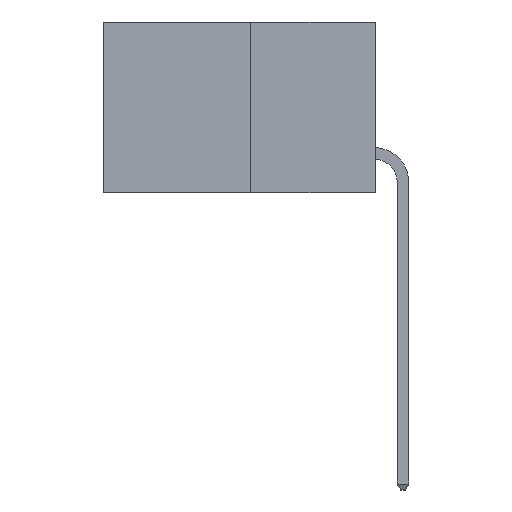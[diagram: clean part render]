
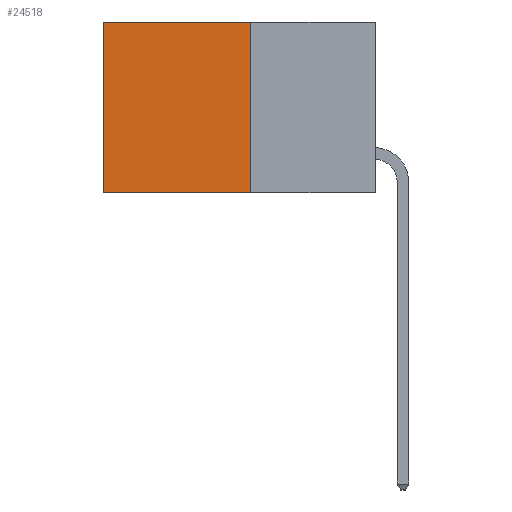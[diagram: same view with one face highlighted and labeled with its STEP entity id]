
A CAD part, left-side view. The second image highlights one B-rep face of the part: STEP entity #24518.
In plain terms, the highlighted planar face has unit normal (-1, 0, 0).
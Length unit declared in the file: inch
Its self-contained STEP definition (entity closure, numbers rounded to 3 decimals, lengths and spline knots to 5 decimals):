
#527 = FACE_OUTER_BOUND ( 'NONE', #14787, .T. ) ;
#1003 = CARTESIAN_POINT ( 'NONE',  ( 0.277, 0.59, -0.37 ) ) ;
#1782 = CARTESIAN_POINT ( 'NONE',  ( 0.277, 0.27, -0.37 ) ) ;
#1924 = CARTESIAN_POINT ( 'NONE',  ( 0.277, 0.27, -0.37 ) ) ;
#3327 = DIRECTION ( 'NONE',  ( 0., 1., 0. ) ) ;
#3908 = EDGE_CURVE ( 'NONE', #16116, #18968, #4880, .T. ) ;
#4880 = LINE ( 'NONE', #24244, #26575 ) ;
#5025 = EDGE_CURVE ( 'NONE', #7314, #5095, #21078, .T. ) ;
#5095 = VERTEX_POINT ( 'NONE', #15826 ) ;
#5703 = PLANE ( 'NONE',  #21764 ) ;
#6089 = ORIENTED_EDGE ( 'NONE', *, *, #5025, .F. ) ;
#6190 = DIRECTION ( 'NONE',  ( 0., 0., -1. ) ) ;
#7314 = VERTEX_POINT ( 'NONE', #1924 ) ;
#9304 = CARTESIAN_POINT ( 'NONE',  ( 0.277, 0.27, -0.37 ) ) ;
#9397 = VECTOR ( 'NONE', #6190, 39.37008 ) ;
#9982 = DIRECTION ( 'NONE',  ( 1., 0., 0. ) ) ;
#10613 = ORIENTED_EDGE ( 'NONE', *, *, #3908, .T. ) ;
#12132 = ORIENTED_EDGE ( 'NONE', *, *, #22088, .F. ) ;
#13594 = VECTOR ( 'NONE', #20131, 39.37008 ) ;
#14787 = EDGE_LOOP ( 'NONE', ( #17951, #6089, #12132, #10613 ) ) ;
#15168 = CARTESIAN_POINT ( 'NONE',  ( 0.277, 0.27, 0. ) ) ;
#15451 = VECTOR ( 'NONE', #19921, 39.37008 ) ;
#15826 = CARTESIAN_POINT ( 'NONE',  ( 0.277, 0.59, -0.37 ) ) ;
#16116 = VERTEX_POINT ( 'NONE', #15168 ) ;
#17603 = CARTESIAN_POINT ( 'NONE',  ( 0.277, 0.59, 0. ) ) ;
#17951 = ORIENTED_EDGE ( 'NONE', *, *, #20519, .T. ) ;
#18968 = VERTEX_POINT ( 'NONE', #17603 ) ;
#19257 = LINE ( 'NONE', #1003, #13594 ) ;
#19921 = DIRECTION ( 'NONE',  ( 0., 1., 0. ) ) ;
#20131 = DIRECTION ( 'NONE',  ( 0., 0., -1. ) ) ;
#20519 = EDGE_CURVE ( 'NONE', #18968, #5095, #19257, .T. ) ;
#21078 = LINE ( 'NONE', #9304, #15451 ) ;
#21764 = AXIS2_PLACEMENT_3D ( 'NONE', #22550, #9982, #24626 ) ;
#22088 = EDGE_CURVE ( 'NONE', #16116, #7314, #26095, .T. ) ;
#22550 = CARTESIAN_POINT ( 'NONE',  ( 0.277, 0.27, -0.37 ) ) ;
#24244 = CARTESIAN_POINT ( 'NONE',  ( 0.277, 0.27, 0. ) ) ;
#24518 = ADVANCED_FACE ( 'NONE', ( #527 ), #5703, .F. ) ;
#24626 = DIRECTION ( 'NONE',  ( 0., 0., -1. ) ) ;
#26095 = LINE ( 'NONE', #1782, #9397 ) ;
#26575 = VECTOR ( 'NONE', #3327, 39.37008 ) ;
